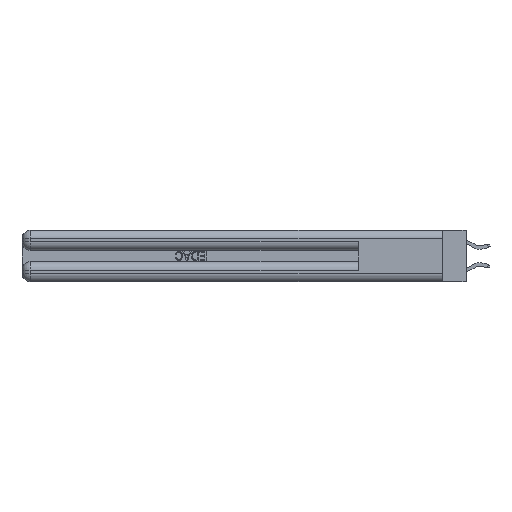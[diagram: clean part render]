
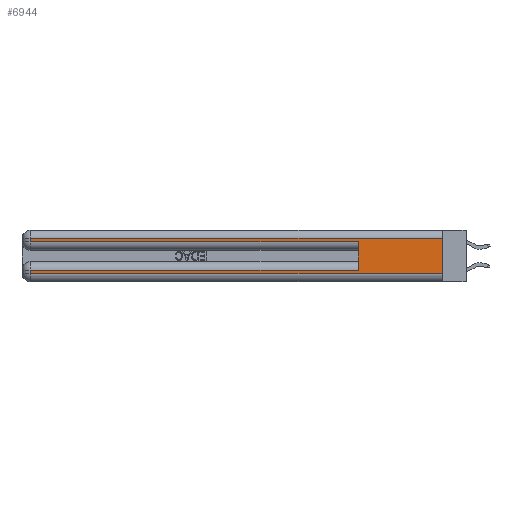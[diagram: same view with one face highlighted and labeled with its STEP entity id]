
A CAD part, left-side view. The second image highlights one B-rep face of the part: STEP entity #6944.
In plain terms, the highlighted planar face has unit normal (-1, 0, 0).
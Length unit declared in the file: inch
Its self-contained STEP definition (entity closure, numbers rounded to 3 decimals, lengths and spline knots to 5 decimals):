
#156 = DIRECTION ( 'NONE',  ( 0., -1., 0. ) ) ;
#876 = DIRECTION ( 'NONE',  ( 0., 0., -1. ) ) ;
#1359 = DIRECTION ( 'NONE',  ( 0., 0., -1. ) ) ;
#1798 = DIRECTION ( 'NONE',  ( 0., -1., 0. ) ) ;
#2302 = VECTOR ( 'NONE', #9214, 39.37008 ) ;
#2755 = CARTESIAN_POINT ( 'NONE',  ( 0., 2.94, 0.06 ) ) ;
#2880 = LINE ( 'NONE', #18467, #21149 ) ;
#3050 = ORIENTED_EDGE ( 'NONE', *, *, #4479, .T. ) ;
#3706 = VERTEX_POINT ( 'NONE', #13681 ) ;
#4336 = CARTESIAN_POINT ( 'NONE',  ( 0., 2.94, 0.085 ) ) ;
#4387 = CARTESIAN_POINT ( 'NONE',  ( 0., 0.6, 0.085 ) ) ;
#4479 = EDGE_CURVE ( 'NONE', #11019, #5893, #17838, .T. ) ;
#5062 = EDGE_CURVE ( 'NONE', #5893, #3706, #2880, .T. ) ;
#5719 = ORIENTED_EDGE ( 'NONE', *, *, #17704, .T. ) ;
#5893 = VERTEX_POINT ( 'NONE', #12411 ) ;
#6912 = LINE ( 'NONE', #16705, #13244 ) ;
#6944 = ADVANCED_FACE ( 'NONE', ( #29634 ), #9868, .F. ) ;
#7388 = VERTEX_POINT ( 'NONE', #4387 ) ;
#9214 = DIRECTION ( 'NONE',  ( 0., 1., 0. ) ) ;
#9362 = DIRECTION ( 'NONE',  ( 0., 0., -1. ) ) ;
#9868 = PLANE ( 'NONE',  #28796 ) ;
#10821 = VECTOR ( 'NONE', #13037, 39.37008 ) ;
#10869 = CARTESIAN_POINT ( 'NONE',  ( 0., 0., 0.37 ) ) ;
#11019 = VERTEX_POINT ( 'NONE', #15593 ) ;
#11768 = CARTESIAN_POINT ( 'NONE',  ( 0., 2.94, 0.37 ) ) ;
#12091 = CARTESIAN_POINT ( 'NONE',  ( 0., 0., 0.06 ) ) ;
#12265 = DIRECTION ( 'NONE',  ( 1., 0., 0. ) ) ;
#12411 = CARTESIAN_POINT ( 'NONE',  ( 0., 2.94, 0.285 ) ) ;
#12921 = ORIENTED_EDGE ( 'NONE', *, *, #27998, .T. ) ;
#12931 = LINE ( 'NONE', #10869, #24828 ) ;
#13037 = DIRECTION ( 'NONE',  ( 0., 0., 1. ) ) ;
#13244 = VECTOR ( 'NONE', #28608, 39.37008 ) ;
#13262 = ORIENTED_EDGE ( 'NONE', *, *, #15735, .T. ) ;
#13681 = CARTESIAN_POINT ( 'NONE',  ( 0., 0.6, 0.285 ) ) ;
#15263 = LINE ( 'NONE', #12091, #27198 ) ;
#15282 = CARTESIAN_POINT ( 'NONE',  ( 0., 0., 0.31 ) ) ;
#15593 = CARTESIAN_POINT ( 'NONE',  ( 0., 2.94, 0.31 ) ) ;
#15735 = EDGE_CURVE ( 'NONE', #26590, #18586, #15854, .T. ) ;
#15854 = LINE ( 'NONE', #27053, #21417 ) ;
#16024 = EDGE_CURVE ( 'NONE', #25027, #11019, #6912, .T. ) ;
#16490 = ORIENTED_EDGE ( 'NONE', *, *, #27674, .F. ) ;
#16705 = CARTESIAN_POINT ( 'NONE',  ( 0., 0., 0.31 ) ) ;
#17092 = VECTOR ( 'NONE', #9362, 39.37008 ) ;
#17129 = LINE ( 'NONE', #24889, #10821 ) ;
#17704 = EDGE_CURVE ( 'NONE', #7388, #26590, #21297, .T. ) ;
#17838 = LINE ( 'NONE', #11768, #17092 ) ;
#18467 = CARTESIAN_POINT ( 'NONE',  ( 0., 0., 0.285 ) ) ;
#18586 = VERTEX_POINT ( 'NONE', #2755 ) ;
#19246 = ORIENTED_EDGE ( 'NONE', *, *, #5062, .T. ) ;
#19294 = CARTESIAN_POINT ( 'NONE',  ( 0., 0., 0.37 ) ) ;
#20233 = ORIENTED_EDGE ( 'NONE', *, *, #22771, .F. ) ;
#21149 = VECTOR ( 'NONE', #1798, 39.37008 ) ;
#21297 = LINE ( 'NONE', #25855, #2302 ) ;
#21417 = VECTOR ( 'NONE', #876, 39.37008 ) ;
#22196 = ORIENTED_EDGE ( 'NONE', *, *, #16024, .T. ) ;
#22771 = EDGE_CURVE ( 'NONE', #25027, #23565, #12931, .T. ) ;
#23565 = VERTEX_POINT ( 'NONE', #30301 ) ;
#24828 = VECTOR ( 'NONE', #1359, 39.37008 ) ;
#24889 = CARTESIAN_POINT ( 'NONE',  ( 0., 0.6, 0.145 ) ) ;
#25027 = VERTEX_POINT ( 'NONE', #15282 ) ;
#25855 = CARTESIAN_POINT ( 'NONE',  ( 0., 0., 0.085 ) ) ;
#26590 = VERTEX_POINT ( 'NONE', #4336 ) ;
#27053 = CARTESIAN_POINT ( 'NONE',  ( 0., 2.94, 0.37 ) ) ;
#27198 = VECTOR ( 'NONE', #156, 39.37008 ) ;
#27674 = EDGE_CURVE ( 'NONE', #7388, #3706, #17129, .T. ) ;
#27998 = EDGE_CURVE ( 'NONE', #18586, #23565, #15263, .T. ) ;
#28608 = DIRECTION ( 'NONE',  ( 0., 1., 0. ) ) ;
#28796 = AXIS2_PLACEMENT_3D ( 'NONE', #19294, #12265, #28921 ) ;
#28921 = DIRECTION ( 'NONE',  ( 0., 0., -1. ) ) ;
#29634 = FACE_OUTER_BOUND ( 'NONE', #30422, .T. ) ;
#30301 = CARTESIAN_POINT ( 'NONE',  ( 0., 0., 0.06 ) ) ;
#30422 = EDGE_LOOP ( 'NONE', ( #20233, #22196, #3050, #19246, #16490, #5719, #13262, #12921 ) ) ;
